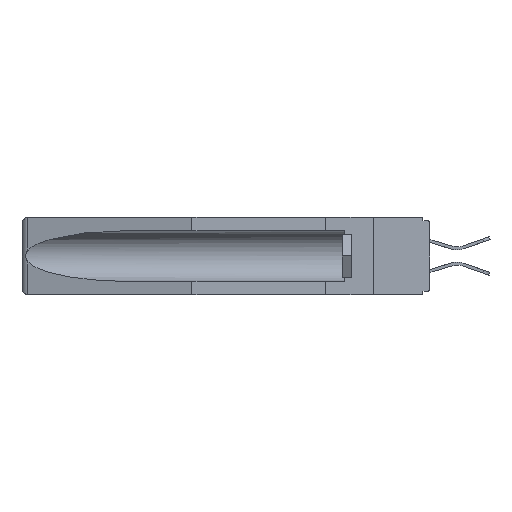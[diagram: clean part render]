
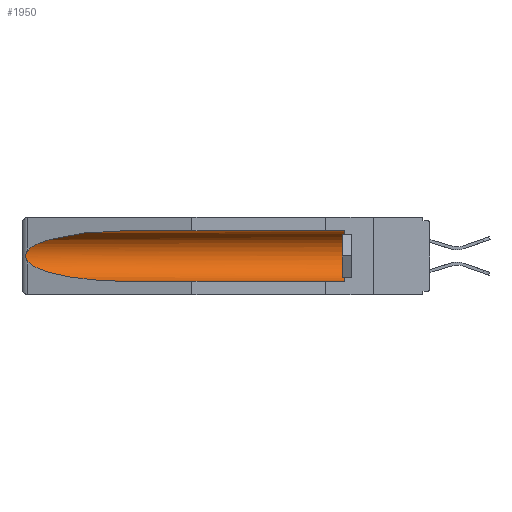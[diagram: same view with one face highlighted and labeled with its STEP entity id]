
A CAD part, left-side view. The second image highlights one B-rep face of the part: STEP entity #1950.
In plain terms, the highlighted cylindrical face has radius 2.857 mm (diameter 5.715 mm), a partial arc.
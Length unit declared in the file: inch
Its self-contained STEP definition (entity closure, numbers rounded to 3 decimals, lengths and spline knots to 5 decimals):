
#885 = CARTESIAN_POINT ( 'NONE',  ( 0.2675, 1.53308, -0.17534 ) ) ;
#965 = CARTESIAN_POINT ( 'NONE',  ( 0.26655, 1.53094, -0.18657 ) ) ;
#1126 = CARTESIAN_POINT ( 'NONE',  ( 0.26537, 1.52718, -0.14972 ) ) ;
#1191 = LINE ( 'NONE', #3626, #3301 ) ;
#1212 = CARTESIAN_POINT ( 'NONE',  ( 0.155, 1.07973, -0.059 ) ) ;
#1329 = CARTESIAN_POINT ( 'NONE',  ( 0.155, 1.07973, -0.059 ) ) ;
#1720 = CARTESIAN_POINT ( 'NONE',  ( 0.155, -0.30754, -0.284 ) ) ;
#1758 = EDGE_CURVE ( 'NONE', #23990, #21007, #12964, .T. ) ;
#1950 = ADVANCED_FACE ( 'NONE', ( #11796 ), #8556, .F. ) ;
#3301 = VECTOR ( 'NONE', #16836, 39.37008 ) ;
#3541 = ORIENTED_EDGE ( 'NONE', *, *, #24116, .T. ) ;
#3626 = CARTESIAN_POINT ( 'NONE',  ( 0.155, -0.30754, -0.059 ) ) ;
#3790 = CARTESIAN_POINT ( 'NONE',  ( 0.21114, 1.30732, -0.284 ) ) ;
#3876 = CARTESIAN_POINT ( 'NONE',  ( 0.155, 1.07973, -0.284 ) ) ;
#3898 = AXIS2_PLACEMENT_3D ( 'NONE', #17321, #23350, #15897 ) ;
#4583 = CARTESIAN_POINT ( 'NONE',  ( 0.26537, 1.52718, -0.14972 ) ) ;
#4925 = DIRECTION ( 'NONE',  ( 0., 0., 1. ) ) ;
#5821 = ORIENTED_EDGE ( 'NONE', *, *, #23066, .T. ) ;
#5992 = VERTEX_POINT ( 'NONE', #1329 ) ;
#6768 = B_SPLINE_CURVE_WITH_KNOTS ( 'NONE', 3,
 ( #1126, #21972, #12298, #21647, #12216, #885, #19808, #965, #19838, #8557 ),
 .UNSPECIFIED., .F., .F.,
 ( 4, 2, 2, 2, 4 ),
 ( 0., 0.00029, 0.00058, 0.00087, 0.00117 ),
 .UNSPECIFIED. ) ;
#7036 = EDGE_CURVE ( 'NONE', #15816, #23990, #6768, .T. ) ;
#7170 = DIRECTION ( 'NONE',  ( 0., 1., 0. ) ) ;
#7666 = CARTESIAN_POINT ( 'NONE',  ( 0.155, 0.126, -0.059 ) ) ;
#8556 = CYLINDRICAL_SURFACE ( 'NONE', #24309, 0.1125 ) ;
#8557 = CARTESIAN_POINT ( 'NONE',  ( 0.26537, 1.52718, -0.19328 ) ) ;
#8664 = ORIENTED_EDGE ( 'NONE', *, *, #1758, .T. ) ;
#8675 = CIRCLE ( 'NONE', #3898, 0.1125 ) ;
#8932 = CARTESIAN_POINT ( 'NONE',  ( 0.26537, 1.52718, -0.19328 ) ) ;
#9705 = CARTESIAN_POINT ( 'NONE',  ( 0.25451, 1.48313, -0.24835 ) ) ;
#9861 = CARTESIAN_POINT ( 'NONE',  ( 0.155, 1.07973, -0.284 ) ) ;
#10392 = EDGE_LOOP ( 'NONE', ( #24285, #10507, #8664, #21194, #5821, #3541 ) ) ;
#10507 = ORIENTED_EDGE ( 'NONE', *, *, #7036, .T. ) ;
#10806 = CARTESIAN_POINT ( 'NONE',  ( 0.26537, 1.52718, -0.14972 ) ) ;
#11796 = FACE_OUTER_BOUND ( 'NONE', #10392, .T. ) ;
#12216 = CARTESIAN_POINT ( 'NONE',  ( 0.2675, 1.53308, -0.16763 ) ) ;
#12298 = CARTESIAN_POINT ( 'NONE',  ( 0.26654, 1.53092, -0.15636 ) ) ;
#12582 = LINE ( 'NONE', #1720, #17341 ) ;
#12964 =( BOUNDED_CURVE ( )  B_SPLINE_CURVE ( 3, ( #21005, #9705, #3790, #3876 ),
 .UNSPECIFIED., .F., .F. ) 
 B_SPLINE_CURVE_WITH_KNOTS ( ( 4, 4 ),
 ( 0.1948, 1.5708 ),
 .UNSPECIFIED. ) 
 CURVE ( )  GEOMETRIC_REPRESENTATION_ITEM ( )  RATIONAL_B_SPLINE_CURVE ( ( 1., 0.848, 0.848, 1. ) ) 
 REPRESENTATION_ITEM ( '' )  );
#15603 = EDGE_CURVE ( 'NONE', #5992, #15816, #20704, .T. ) ;
#15816 = VERTEX_POINT ( 'NONE', #4583 ) ;
#15897 = DIRECTION ( 'NONE',  ( 0., 0., 1. ) ) ;
#16836 = DIRECTION ( 'NONE',  ( 0., 1., 0. ) ) ;
#17321 = CARTESIAN_POINT ( 'NONE',  ( 0.155, 0.126, -0.1715 ) ) ;
#17341 = VECTOR ( 'NONE', #7170, 39.37008 ) ;
#19586 = DIRECTION ( 'NONE',  ( 0., 1., 0. ) ) ;
#19808 = CARTESIAN_POINT ( 'NONE',  ( 0.2673, 1.53269, -0.17917 ) ) ;
#19838 = CARTESIAN_POINT ( 'NONE',  ( 0.26597, 1.5296, -0.19026 ) ) ;
#20024 = CARTESIAN_POINT ( 'NONE',  ( 0.155, 0.126, -0.284 ) ) ;
#20220 = CARTESIAN_POINT ( 'NONE',  ( 0.21114, 1.30732, -0.059 ) ) ;
#20704 =( BOUNDED_CURVE ( )  B_SPLINE_CURVE ( 3, ( #1212, #20220, #22146, #10806 ),
 .UNSPECIFIED., .F., .F. ) 
 B_SPLINE_CURVE_WITH_KNOTS ( ( 4, 4 ),
 ( 4.71239, 6.08839 ),
 .UNSPECIFIED. ) 
 CURVE ( )  GEOMETRIC_REPRESENTATION_ITEM ( )  RATIONAL_B_SPLINE_CURVE ( ( 1., 0.848, 0.848, 1. ) ) 
 REPRESENTATION_ITEM ( '' )  );
#21005 = CARTESIAN_POINT ( 'NONE',  ( 0.26537, 1.52718, -0.19328 ) ) ;
#21007 = VERTEX_POINT ( 'NONE', #9861 ) ;
#21194 = ORIENTED_EDGE ( 'NONE', *, *, #22160, .F. ) ;
#21424 = CARTESIAN_POINT ( 'NONE',  ( 0.155, -0.30754, -0.1715 ) ) ;
#21647 = CARTESIAN_POINT ( 'NONE',  ( 0.2673, 1.5327, -0.16383 ) ) ;
#21972 = CARTESIAN_POINT ( 'NONE',  ( 0.26597, 1.52961, -0.15275 ) ) ;
#22146 = CARTESIAN_POINT ( 'NONE',  ( 0.25451, 1.48313, -0.09465 ) ) ;
#22160 = EDGE_CURVE ( 'NONE', #23586, #21007, #12582, .T. ) ;
#22319 = VERTEX_POINT ( 'NONE', #7666 ) ;
#23066 = EDGE_CURVE ( 'NONE', #23586, #22319, #8675, .T. ) ;
#23350 = DIRECTION ( 'NONE',  ( 0., -1., 0. ) ) ;
#23586 = VERTEX_POINT ( 'NONE', #20024 ) ;
#23990 = VERTEX_POINT ( 'NONE', #8932 ) ;
#24116 = EDGE_CURVE ( 'NONE', #22319, #5992, #1191, .T. ) ;
#24285 = ORIENTED_EDGE ( 'NONE', *, *, #15603, .T. ) ;
#24309 = AXIS2_PLACEMENT_3D ( 'NONE', #21424, #19586, #4925 ) ;
